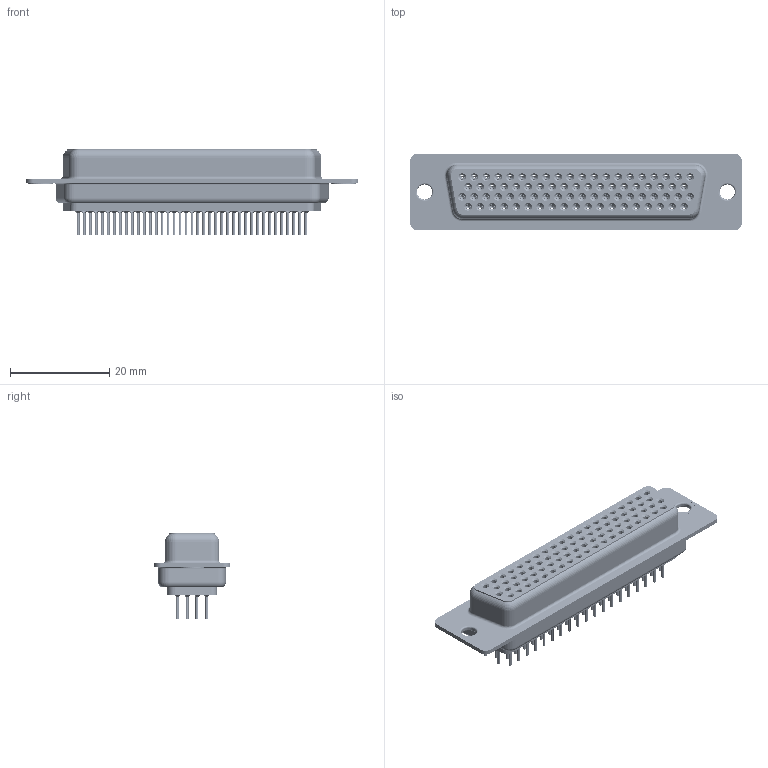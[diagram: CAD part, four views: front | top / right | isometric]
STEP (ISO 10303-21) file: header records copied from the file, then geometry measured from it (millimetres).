
FILE_DESCRIPTION (( 'STEP AP203' ), '1' );
FILE_NAME ('638-078-630-041.STEP', '2020-07-20T04:25:29', ( '' ), ( '' ), 'SwSTEP 2.0', 'SolidWorks 2020', '' );
FILE_SCHEMA (( 'CONFIG_CONTROL_DESIGN' ));
Length unit declared in the file: millimetre
Products named in the file (9): 638 Contact Row 2_30; 638 Contact Row 78_30; 638 Contact Row 3_30; 638 Shell Rear_78 Contacts; 638 Shell Front_78 Contacts; 638-078-630-041; 638 Housing_78 Contacts; 638 Contact Row 1_30; 638 Thru Hole Rivet
Assembly tree (83 placements, depth 2):
  638-078-630-041
    638 Housing_78 Contacts
    638 Shell Front_78 Contacts
    638 Shell Rear_78 Contacts
    638 Contact Row 1_30  x19
    638 Contact Row 2_30  x20
    638 Contact Row 3_30  x19
    638 Contact Row 78_30  x20
    638 Thru Hole Rivet  x2
Bounding box: 67 x 15.4 x 17.3 mm (x, y, z)
Volume: 5797.1 mm3; surface area: 20377.7 mm2
Topology: 83 solids, 83 shells, 10159 faces, 25835 edges, 16009 vertices
Faces by surface type: cylinder 2695, plane 2485, torus 2133, bspline 1560, cone 1286
Entity records: 55963 total; most frequent: CARTESIAN_POINT 13099, DIRECTION 8995, ORIENTED_EDGE 7826, EDGE_CURVE 3913, AXIS2_PLACEMENT_3D 3820, VERTEX_POINT 2475, CIRCLE 2117, EDGE_LOOP 2110
